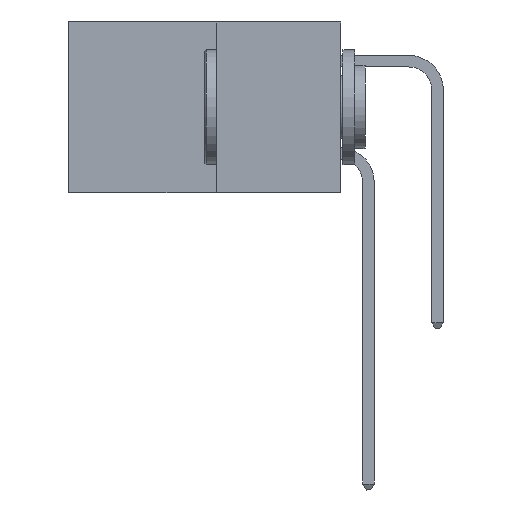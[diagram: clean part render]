
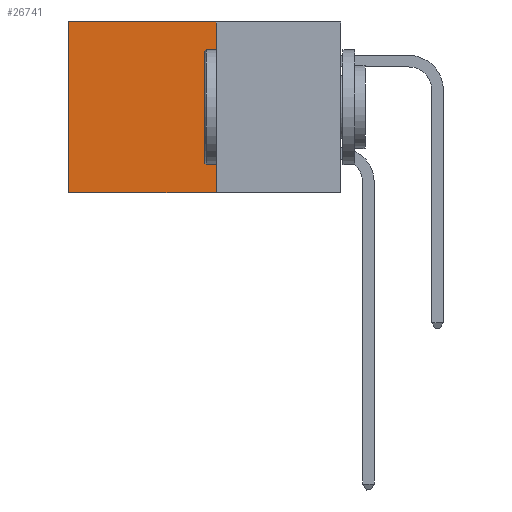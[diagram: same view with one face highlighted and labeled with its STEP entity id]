
A CAD part, left-side view. The second image highlights one B-rep face of the part: STEP entity #26741.
In plain terms, the highlighted planar face has unit normal (-1, 0, 0).
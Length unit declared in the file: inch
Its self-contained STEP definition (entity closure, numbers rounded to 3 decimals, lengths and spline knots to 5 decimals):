
#616 = DIRECTION ( 'NONE',  ( 0., 1., 0. ) ) ;
#803 = CARTESIAN_POINT ( 'NONE',  ( 0.277, 0.27, -0.37 ) ) ;
#943 = CARTESIAN_POINT ( 'NONE',  ( 0.277, 0.27, -0.37 ) ) ;
#3246 = PLANE ( 'NONE',  #18339 ) ;
#5510 = VERTEX_POINT ( 'NONE', #27838 ) ;
#5644 = EDGE_CURVE ( 'NONE', #5510, #23302, #7708, .T. ) ;
#7480 = CARTESIAN_POINT ( 'NONE',  ( 0.277, 0.59, -0.37 ) ) ;
#7641 = VECTOR ( 'NONE', #616, 39.37008 ) ;
#7708 = LINE ( 'NONE', #18561, #21476 ) ;
#8668 = ORIENTED_EDGE ( 'NONE', *, *, #5644, .F. ) ;
#9319 = FACE_OUTER_BOUND ( 'NONE', #21879, .T. ) ;
#10940 = DIRECTION ( 'NONE',  ( 0., 0., -1. ) ) ;
#11273 = VECTOR ( 'NONE', #26277, 39.37008 ) ;
#12193 = EDGE_CURVE ( 'NONE', #23302, #17106, #14175, .T. ) ;
#12325 = ORIENTED_EDGE ( 'NONE', *, *, #30408, .T. ) ;
#14175 = LINE ( 'NONE', #29724, #7641 ) ;
#14965 = VECTOR ( 'NONE', #10940, 39.37008 ) ;
#17106 = VERTEX_POINT ( 'NONE', #7480 ) ;
#17538 = CARTESIAN_POINT ( 'NONE',  ( 0.277, 0.59, 0. ) ) ;
#17982 = DIRECTION ( 'NONE',  ( 0., 0., -1. ) ) ;
#18339 = AXIS2_PLACEMENT_3D ( 'NONE', #803, #22642, #20358 ) ;
#18475 = LINE ( 'NONE', #23850, #11273 ) ;
#18561 = CARTESIAN_POINT ( 'NONE',  ( 0.277, 0.27, -0.37 ) ) ;
#18662 = VERTEX_POINT ( 'NONE', #17538 ) ;
#20358 = DIRECTION ( 'NONE',  ( 0., 0., -1. ) ) ;
#21476 = VECTOR ( 'NONE', #17982, 39.37008 ) ;
#21879 = EDGE_LOOP ( 'NONE', ( #12325, #25767, #8668, #30435 ) ) ;
#22642 = DIRECTION ( 'NONE',  ( 1., 0., 0. ) ) ;
#23302 = VERTEX_POINT ( 'NONE', #943 ) ;
#23850 = CARTESIAN_POINT ( 'NONE',  ( 0.277, 0.27, 0. ) ) ;
#25432 = CARTESIAN_POINT ( 'NONE',  ( 0.277, 0.59, -0.37 ) ) ;
#25767 = ORIENTED_EDGE ( 'NONE', *, *, #12193, .F. ) ;
#26277 = DIRECTION ( 'NONE',  ( 0., 1., 0. ) ) ;
#26298 = LINE ( 'NONE', #25432, #14965 ) ;
#26741 = ADVANCED_FACE ( 'NONE', ( #9319 ), #3246, .F. ) ;
#27838 = CARTESIAN_POINT ( 'NONE',  ( 0.277, 0.27, 0. ) ) ;
#29678 = EDGE_CURVE ( 'NONE', #5510, #18662, #18475, .T. ) ;
#29724 = CARTESIAN_POINT ( 'NONE',  ( 0.277, 0.27, -0.37 ) ) ;
#30408 = EDGE_CURVE ( 'NONE', #18662, #17106, #26298, .T. ) ;
#30435 = ORIENTED_EDGE ( 'NONE', *, *, #29678, .T. ) ;
